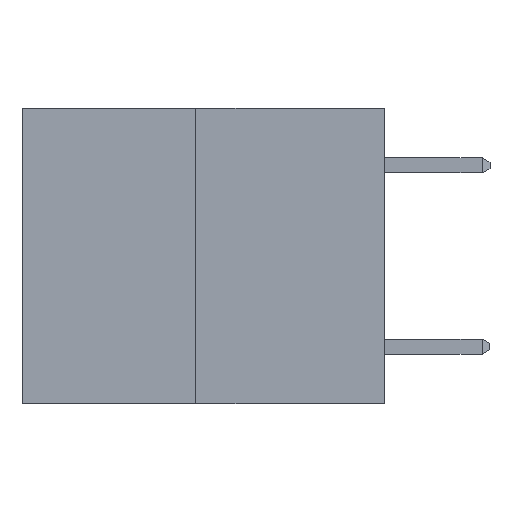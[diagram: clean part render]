
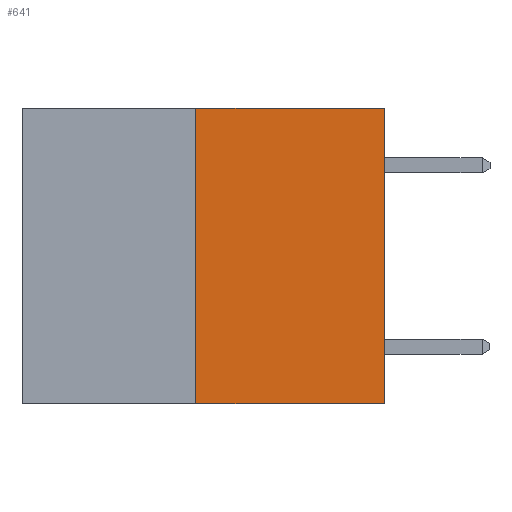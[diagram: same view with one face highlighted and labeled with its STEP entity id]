
A CAD part, left-side view. The second image highlights one B-rep face of the part: STEP entity #641.
In plain terms, the highlighted planar face has unit normal (-1, 0, 0).
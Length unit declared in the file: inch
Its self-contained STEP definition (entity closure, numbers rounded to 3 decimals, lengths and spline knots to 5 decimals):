
#169 = VERTEX_POINT ( 'NONE', #13322 ) ;
#218 = CARTESIAN_POINT ( 'NONE',  ( 0., 0.6, 0. ) ) ;
#314 = EDGE_CURVE ( 'NONE', #13229, #3216, #768, .T. ) ;
#326 = ORIENTED_EDGE ( 'NONE', *, *, #314, .T. ) ;
#641 = ADVANCED_FACE ( 'NONE', ( #7536 ), #2682, .F. ) ;
#724 = EDGE_CURVE ( 'NONE', #3216, #4491, #5780, .T. ) ;
#768 = LINE ( 'NONE', #11921, #13924 ) ;
#1497 = CARTESIAN_POINT ( 'NONE',  ( 0., 0.312, -0.49 ) ) ;
#1631 = AXIS2_PLACEMENT_3D ( 'NONE', #12570, #6377, #14992 ) ;
#2526 = VECTOR ( 'NONE', #2988, 39.37008 ) ;
#2682 = PLANE ( 'NONE',  #1631 ) ;
#2988 = DIRECTION ( 'NONE',  ( 0., 0., 1. ) ) ;
#3216 = VERTEX_POINT ( 'NONE', #13659 ) ;
#4491 = VERTEX_POINT ( 'NONE', #11772 ) ;
#5780 = LINE ( 'NONE', #12983, #2526 ) ;
#6377 = DIRECTION ( 'NONE',  ( 1., 0., 0. ) ) ;
#6410 = DIRECTION ( 'NONE',  ( 0., -1., 0. ) ) ;
#7111 = DIRECTION ( 'NONE',  ( 0., -1., 0. ) ) ;
#7536 = FACE_OUTER_BOUND ( 'NONE', #13150, .T. ) ;
#7551 = ORIENTED_EDGE ( 'NONE', *, *, #724, .T. ) ;
#8703 = EDGE_CURVE ( 'NONE', #13229, #169, #14223, .T. ) ;
#10763 = ORIENTED_EDGE ( 'NONE', *, *, #8703, .F. ) ;
#11146 = EDGE_CURVE ( 'NONE', #169, #4491, #13397, .T. ) ;
#11772 = CARTESIAN_POINT ( 'NONE',  ( 0., 0., 0. ) ) ;
#11921 = CARTESIAN_POINT ( 'NONE',  ( 0., 0.6, -0.49 ) ) ;
#12570 = CARTESIAN_POINT ( 'NONE',  ( 0., 0.6, 0. ) ) ;
#12983 = CARTESIAN_POINT ( 'NONE',  ( 0., 0., 0. ) ) ;
#13150 = EDGE_LOOP ( 'NONE', ( #10763, #326, #7551, #15636 ) ) ;
#13229 = VERTEX_POINT ( 'NONE', #13963 ) ;
#13322 = CARTESIAN_POINT ( 'NONE',  ( 0., 0.312, 0. ) ) ;
#13381 = VECTOR ( 'NONE', #6410, 39.37008 ) ;
#13397 = LINE ( 'NONE', #218, #13381 ) ;
#13659 = CARTESIAN_POINT ( 'NONE',  ( 0., 0., -0.49 ) ) ;
#13867 = DIRECTION ( 'NONE',  ( 0., 0., 1. ) ) ;
#13924 = VECTOR ( 'NONE', #7111, 39.37008 ) ;
#13963 = CARTESIAN_POINT ( 'NONE',  ( 0., 0.312, -0.49 ) ) ;
#14223 = LINE ( 'NONE', #1497, #15158 ) ;
#14992 = DIRECTION ( 'NONE',  ( 0., 0., -1. ) ) ;
#15158 = VECTOR ( 'NONE', #13867, 39.37008 ) ;
#15636 = ORIENTED_EDGE ( 'NONE', *, *, #11146, .F. ) ;
